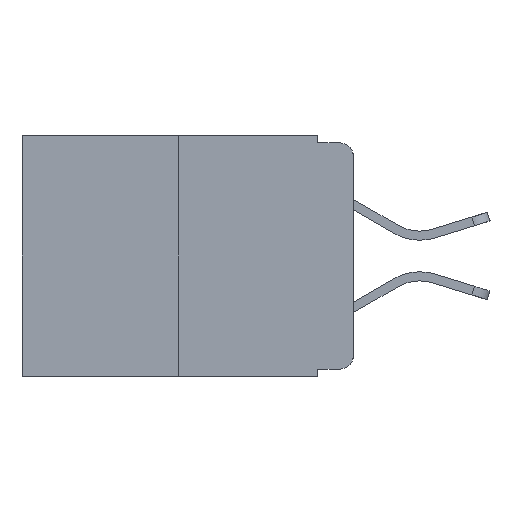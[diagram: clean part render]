
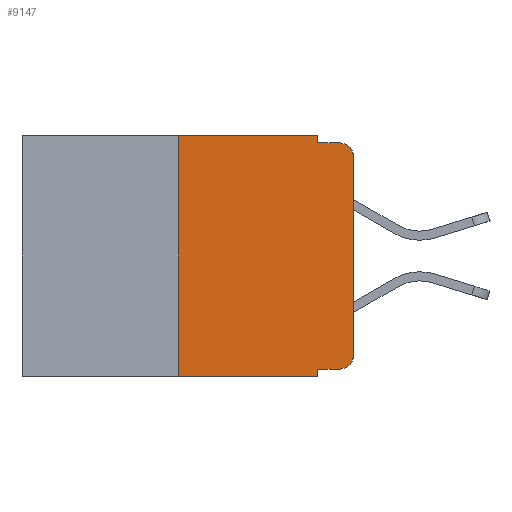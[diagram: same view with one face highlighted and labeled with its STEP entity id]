
A CAD part, left-side view. The second image highlights one B-rep face of the part: STEP entity #9147.
In plain terms, the highlighted planar face has unit normal (-1, 0, 0).
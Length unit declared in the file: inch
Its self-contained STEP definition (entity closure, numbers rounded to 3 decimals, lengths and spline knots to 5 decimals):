
#48 = CARTESIAN_POINT ( 'NONE',  ( 0., 0.25, 0. ) ) ;
#61 = VECTOR ( 'NONE', #5522, 39.37008 ) ;
#162 = VECTOR ( 'NONE', #9563, 39.37008 ) ;
#213 = ORIENTED_EDGE ( 'NONE', *, *, #7997, .T. ) ;
#235 = VERTEX_POINT ( 'NONE', #8551 ) ;
#325 = ORIENTED_EDGE ( 'NONE', *, *, #1370, .T. ) ;
#357 = VERTEX_POINT ( 'NONE', #7543 ) ;
#489 = CARTESIAN_POINT ( 'NONE',  ( 0., 0.473, 0. ) ) ;
#568 = ORIENTED_EDGE ( 'NONE', *, *, #2848, .F. ) ;
#703 = VERTEX_POINT ( 'NONE', #6758 ) ;
#803 = PLANE ( 'NONE',  #6244 ) ;
#918 = DIRECTION ( 'NONE',  ( 0., 0., 1. ) ) ;
#931 = EDGE_CURVE ( 'NONE', #9589, #9840, #4117, .T. ) ;
#936 = DIRECTION ( 'NONE',  ( 0., 0., 1. ) ) ;
#1010 = CARTESIAN_POINT ( 'NONE',  ( 0., 0.051, -0.01 ) ) ;
#1042 = CARTESIAN_POINT ( 'NONE',  ( 0., 0.02, -0.01 ) ) ;
#1124 = CARTESIAN_POINT ( 'NONE',  ( 0., 0.25, 0. ) ) ;
#1236 = VERTEX_POINT ( 'NONE', #1010 ) ;
#1370 = EDGE_CURVE ( 'NONE', #6781, #357, #10963, .T. ) ;
#1538 = VECTOR ( 'NONE', #918, 39.37008 ) ;
#1539 = EDGE_CURVE ( 'NONE', #235, #1236, #6887, .T. ) ;
#1561 = LINE ( 'NONE', #489, #10684 ) ;
#1600 = VECTOR ( 'NONE', #936, 39.37008 ) ;
#2613 = CARTESIAN_POINT ( 'NONE',  ( 0., 0.051, 0. ) ) ;
#2646 = VERTEX_POINT ( 'NONE', #1042 ) ;
#2848 = EDGE_CURVE ( 'NONE', #703, #11346, #9915, .T. ) ;
#3451 = CARTESIAN_POINT ( 'NONE',  ( 0., 0.051, -0.01 ) ) ;
#3518 = VECTOR ( 'NONE', #4231, 39.37008 ) ;
#3903 = AXIS2_PLACEMENT_3D ( 'NONE', #9084, #11155, #5190 ) ;
#4058 = LINE ( 'NONE', #4656, #1538 ) ;
#4117 = LINE ( 'NONE', #1124, #1600 ) ;
#4119 = LINE ( 'NONE', #8096, #3518 ) ;
#4231 = DIRECTION ( 'NONE',  ( 0., -1., 0. ) ) ;
#4547 = VECTOR ( 'NONE', #6161, 39.37008 ) ;
#4581 = DIRECTION ( 'NONE',  ( 0., 0., -1. ) ) ;
#4609 = CARTESIAN_POINT ( 'NONE',  ( 0., 0.473, -0.343 ) ) ;
#4656 = CARTESIAN_POINT ( 'NONE',  ( 0., 0., 0. ) ) ;
#4745 = EDGE_CURVE ( 'NONE', #703, #6781, #4119, .T. ) ;
#4781 = CARTESIAN_POINT ( 'NONE',  ( 0., 0.051, 0. ) ) ;
#4851 = LINE ( 'NONE', #3451, #4547 ) ;
#5036 = LINE ( 'NONE', #4609, #61 ) ;
#5085 = ORIENTED_EDGE ( 'NONE', *, *, #5535, .F. ) ;
#5190 = DIRECTION ( 'NONE',  ( 0., 0., -1. ) ) ;
#5263 = CARTESIAN_POINT ( 'NONE',  ( 0., 0.25, -0.343 ) ) ;
#5405 = CARTESIAN_POINT ( 'NONE',  ( 0., 0.02, -0.03 ) ) ;
#5522 = DIRECTION ( 'NONE',  ( 0., -1., 0. ) ) ;
#5535 = EDGE_CURVE ( 'NONE', #1236, #2646, #4851, .T. ) ;
#5597 = EDGE_CURVE ( 'NONE', #10400, #2646, #8929, .T. ) ;
#5656 = DIRECTION ( 'NONE',  ( 0., 0., -1. ) ) ;
#6161 = DIRECTION ( 'NONE',  ( 0., -1., 0. ) ) ;
#6244 = AXIS2_PLACEMENT_3D ( 'NONE', #11344, #9762, #4581 ) ;
#6269 = DIRECTION ( 'NONE',  ( 0., 0., -1. ) ) ;
#6304 = ORIENTED_EDGE ( 'NONE', *, *, #10656, .F. ) ;
#6380 = EDGE_LOOP ( 'NONE', ( #213, #11033, #5085, #10160, #6304, #7929, #10441, #568, #8814, #325 ) ) ;
#6758 = CARTESIAN_POINT ( 'NONE',  ( 0., 0.051, -0.333 ) ) ;
#6781 = VERTEX_POINT ( 'NONE', #8970 ) ;
#6887 = LINE ( 'NONE', #2613, #162 ) ;
#7026 = AXIS2_PLACEMENT_3D ( 'NONE', #5405, #11280, #6269 ) ;
#7109 = CARTESIAN_POINT ( 'NONE',  ( 0., 0.051, -0.343 ) ) ;
#7543 = CARTESIAN_POINT ( 'NONE',  ( 0., 0., -0.313 ) ) ;
#7929 = ORIENTED_EDGE ( 'NONE', *, *, #931, .F. ) ;
#7997 = EDGE_CURVE ( 'NONE', #357, #10400, #4058, .T. ) ;
#8096 = CARTESIAN_POINT ( 'NONE',  ( 0., 0.051, -0.333 ) ) ;
#8551 = CARTESIAN_POINT ( 'NONE',  ( 0., 0.051, 0. ) ) ;
#8814 = ORIENTED_EDGE ( 'NONE', *, *, #4745, .T. ) ;
#8929 = CIRCLE ( 'NONE', #7026, 0.02 ) ;
#8970 = CARTESIAN_POINT ( 'NONE',  ( 0., 0.02, -0.333 ) ) ;
#9084 = CARTESIAN_POINT ( 'NONE',  ( 0., 0.02, -0.313 ) ) ;
#9147 = ADVANCED_FACE ( 'NONE', ( #10002 ), #803, .F. ) ;
#9475 = DIRECTION ( 'NONE',  ( 0., -1., 0. ) ) ;
#9563 = DIRECTION ( 'NONE',  ( 0., 0., -1. ) ) ;
#9589 = VERTEX_POINT ( 'NONE', #5263 ) ;
#9652 = VECTOR ( 'NONE', #5656, 39.37008 ) ;
#9762 = DIRECTION ( 'NONE',  ( 1., 0., 0. ) ) ;
#9767 = EDGE_CURVE ( 'NONE', #9589, #11346, #5036, .T. ) ;
#9840 = VERTEX_POINT ( 'NONE', #48 ) ;
#9915 = LINE ( 'NONE', #4781, #9652 ) ;
#10002 = FACE_OUTER_BOUND ( 'NONE', #6380, .T. ) ;
#10160 = ORIENTED_EDGE ( 'NONE', *, *, #1539, .F. ) ;
#10400 = VERTEX_POINT ( 'NONE', #10741 ) ;
#10441 = ORIENTED_EDGE ( 'NONE', *, *, #9767, .T. ) ;
#10656 = EDGE_CURVE ( 'NONE', #9840, #235, #1561, .T. ) ;
#10684 = VECTOR ( 'NONE', #9475, 39.37008 ) ;
#10741 = CARTESIAN_POINT ( 'NONE',  ( 0., 0., -0.03 ) ) ;
#10963 = CIRCLE ( 'NONE', #3903, 0.02 ) ;
#11033 = ORIENTED_EDGE ( 'NONE', *, *, #5597, .T. ) ;
#11155 = DIRECTION ( 'NONE',  ( -1., 0., 0. ) ) ;
#11280 = DIRECTION ( 'NONE',  ( -1., 0., 0. ) ) ;
#11344 = CARTESIAN_POINT ( 'NONE',  ( 0., 0.473, 0. ) ) ;
#11346 = VERTEX_POINT ( 'NONE', #7109 ) ;
